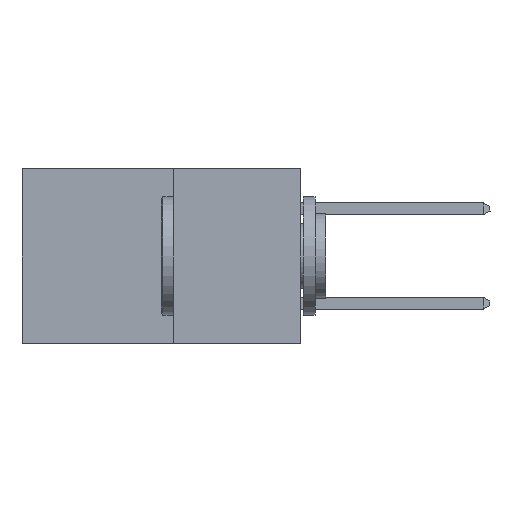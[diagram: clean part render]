
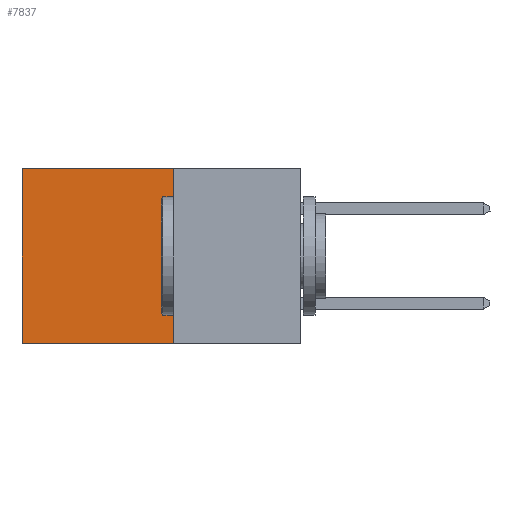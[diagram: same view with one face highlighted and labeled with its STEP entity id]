
A CAD part, left-side view. The second image highlights one B-rep face of the part: STEP entity #7837.
In plain terms, the highlighted planar face has unit normal (-1, 0, 0).
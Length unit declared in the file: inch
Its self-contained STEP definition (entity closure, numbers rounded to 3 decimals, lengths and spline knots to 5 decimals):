
#330 = LINE ( 'NONE', #4251, #12257 ) ;
#1105 = VERTEX_POINT ( 'NONE', #17946 ) ;
#1956 = VERTEX_POINT ( 'NONE', #2860 ) ;
#2162 = ORIENTED_EDGE ( 'NONE', *, *, #25467, .T. ) ;
#2258 = EDGE_CURVE ( 'NONE', #1956, #26211, #330, .T. ) ;
#2860 = CARTESIAN_POINT ( 'NONE',  ( 0.277, 0.27, 0. ) ) ;
#3153 = DIRECTION ( 'NONE',  ( 0., 1., 0. ) ) ;
#4244 = ORIENTED_EDGE ( 'NONE', *, *, #12848, .F. ) ;
#4251 = CARTESIAN_POINT ( 'NONE',  ( 0.277, 0.27, 0. ) ) ;
#4971 = LINE ( 'NONE', #9728, #26522 ) ;
#5026 = CARTESIAN_POINT ( 'NONE',  ( 0.277, 0.27, -0.37 ) ) ;
#7837 = ADVANCED_FACE ( 'NONE', ( #8685 ), #20870, .F. ) ;
#8671 = EDGE_CURVE ( 'NONE', #1956, #15375, #4971, .T. ) ;
#8685 = FACE_OUTER_BOUND ( 'NONE', #26041, .T. ) ;
#9642 = DIRECTION ( 'NONE',  ( 0., 0., -1. ) ) ;
#9728 = CARTESIAN_POINT ( 'NONE',  ( 0.277, 0.27, -0.37 ) ) ;
#10945 = LINE ( 'NONE', #5026, #22640 ) ;
#12257 = VECTOR ( 'NONE', #3153, 39.37008 ) ;
#12848 = EDGE_CURVE ( 'NONE', #15375, #1105, #10945, .T. ) ;
#13618 = CARTESIAN_POINT ( 'NONE',  ( 0.277, 0.27, -0.37 ) ) ;
#14427 = DIRECTION ( 'NONE',  ( 0., 0., -1. ) ) ;
#14774 = LINE ( 'NONE', #26815, #24460 ) ;
#15375 = VERTEX_POINT ( 'NONE', #13618 ) ;
#17036 = ORIENTED_EDGE ( 'NONE', *, *, #2258, .T. ) ;
#17946 = CARTESIAN_POINT ( 'NONE',  ( 0.277, 0.59, -0.37 ) ) ;
#19678 = DIRECTION ( 'NONE',  ( 0., 1., 0. ) ) ;
#20815 = DIRECTION ( 'NONE',  ( 0., 0., -1. ) ) ;
#20844 = DIRECTION ( 'NONE',  ( 1., 0., 0. ) ) ;
#20870 = PLANE ( 'NONE',  #22414 ) ;
#21217 = CARTESIAN_POINT ( 'NONE',  ( 0.277, 0.27, -0.37 ) ) ;
#22414 = AXIS2_PLACEMENT_3D ( 'NONE', #21217, #20844, #20815 ) ;
#22640 = VECTOR ( 'NONE', #19678, 39.37008 ) ;
#24460 = VECTOR ( 'NONE', #14427, 39.37008 ) ;
#24513 = CARTESIAN_POINT ( 'NONE',  ( 0.277, 0.59, 0. ) ) ;
#25467 = EDGE_CURVE ( 'NONE', #26211, #1105, #14774, .T. ) ;
#26041 = EDGE_LOOP ( 'NONE', ( #2162, #4244, #26546, #17036 ) ) ;
#26211 = VERTEX_POINT ( 'NONE', #24513 ) ;
#26522 = VECTOR ( 'NONE', #9642, 39.37008 ) ;
#26546 = ORIENTED_EDGE ( 'NONE', *, *, #8671, .F. ) ;
#26815 = CARTESIAN_POINT ( 'NONE',  ( 0.277, 0.59, -0.37 ) ) ;
